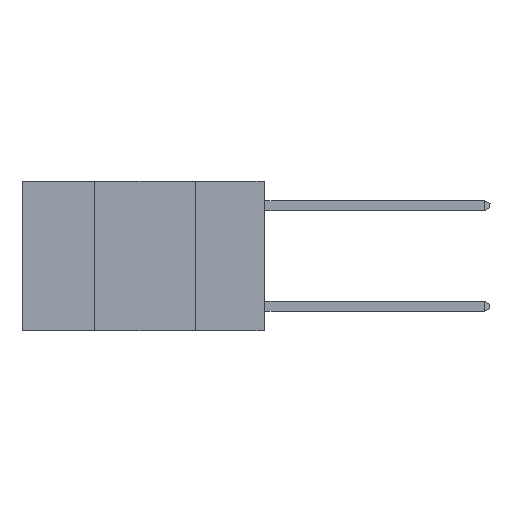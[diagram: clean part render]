
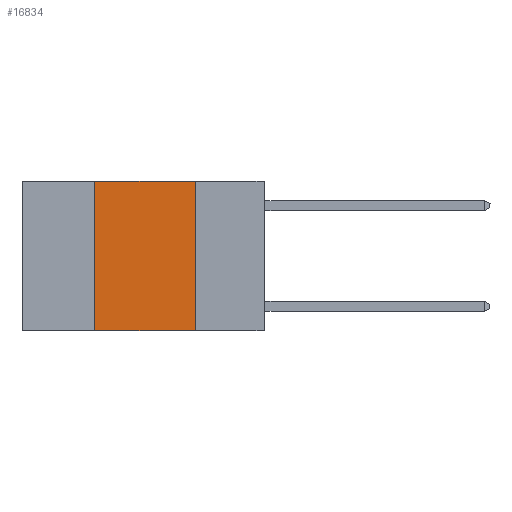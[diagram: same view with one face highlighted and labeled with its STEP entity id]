
A CAD part, left-side view. The second image highlights one B-rep face of the part: STEP entity #16834.
In plain terms, the highlighted planar face has unit normal (-1, 0, 0).
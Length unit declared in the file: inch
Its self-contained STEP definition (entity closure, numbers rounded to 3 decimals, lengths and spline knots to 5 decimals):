
#971 = FACE_OUTER_BOUND ( 'NONE', #15701, .T. ) ;
#1177 = LINE ( 'NONE', #9516, #6439 ) ;
#2124 = DIRECTION ( 'NONE',  ( 0., -1., 0. ) ) ;
#2472 = DIRECTION ( 'NONE',  ( 0., -1., 0. ) ) ;
#2636 = DIRECTION ( 'NONE',  ( 0., 0., -1. ) ) ;
#3166 = EDGE_CURVE ( 'NONE', #16677, #16575, #3607, .T. ) ;
#3607 = LINE ( 'NONE', #14804, #7925 ) ;
#4758 = CARTESIAN_POINT ( 'NONE',  ( 0., 0.42, -0.37 ) ) ;
#5401 = EDGE_CURVE ( 'NONE', #8137, #16677, #17494, .T. ) ;
#6439 = VECTOR ( 'NONE', #2472, 39.37008 ) ;
#7129 = CARTESIAN_POINT ( 'NONE',  ( 0., 0.17, -0.37 ) ) ;
#7298 = EDGE_CURVE ( 'NONE', #8137, #14856, #1177, .T. ) ;
#7925 = VECTOR ( 'NONE', #2124, 39.37008 ) ;
#8137 = VERTEX_POINT ( 'NONE', #4758 ) ;
#9516 = CARTESIAN_POINT ( 'NONE',  ( 0., 0.6, -0.37 ) ) ;
#9656 = PLANE ( 'NONE',  #12131 ) ;
#9667 = EDGE_CURVE ( 'NONE', #16575, #14856, #14982, .T. ) ;
#9756 = DIRECTION ( 'NONE',  ( 1., 0., 0. ) ) ;
#10648 = DIRECTION ( 'NONE',  ( 0., 0., 1. ) ) ;
#12131 = AXIS2_PLACEMENT_3D ( 'NONE', #15304, #9756, #2636 ) ;
#12850 = VECTOR ( 'NONE', #10648, 39.37008 ) ;
#13091 = CARTESIAN_POINT ( 'NONE',  ( 0., 0.17, 0. ) ) ;
#13600 = CARTESIAN_POINT ( 'NONE',  ( 0., 0.17, 0. ) ) ;
#14801 = ORIENTED_EDGE ( 'NONE', *, *, #5401, .F. ) ;
#14804 = CARTESIAN_POINT ( 'NONE',  ( 0., 0.6, 0. ) ) ;
#14856 = VERTEX_POINT ( 'NONE', #7129 ) ;
#14982 = LINE ( 'NONE', #13600, #15071 ) ;
#15071 = VECTOR ( 'NONE', #15258, 39.37008 ) ;
#15258 = DIRECTION ( 'NONE',  ( 0., 0., -1. ) ) ;
#15304 = CARTESIAN_POINT ( 'NONE',  ( 0., 0.6, 0. ) ) ;
#15701 = EDGE_LOOP ( 'NONE', ( #18031, #17391, #14801, #16525 ) ) ;
#16016 = CARTESIAN_POINT ( 'NONE',  ( 0., 0.42, 0. ) ) ;
#16525 = ORIENTED_EDGE ( 'NONE', *, *, #7298, .T. ) ;
#16575 = VERTEX_POINT ( 'NONE', #13091 ) ;
#16677 = VERTEX_POINT ( 'NONE', #17537 ) ;
#16834 = ADVANCED_FACE ( 'NONE', ( #971 ), #9656, .F. ) ;
#17391 = ORIENTED_EDGE ( 'NONE', *, *, #3166, .F. ) ;
#17494 = LINE ( 'NONE', #16016, #12850 ) ;
#17537 = CARTESIAN_POINT ( 'NONE',  ( 0., 0.42, 0. ) ) ;
#18031 = ORIENTED_EDGE ( 'NONE', *, *, #9667, .F. ) ;
